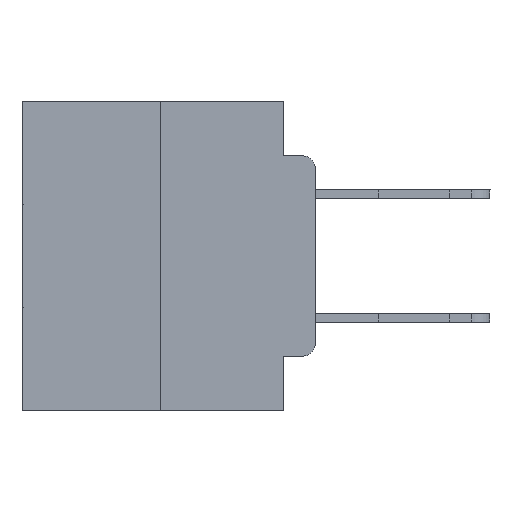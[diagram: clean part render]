
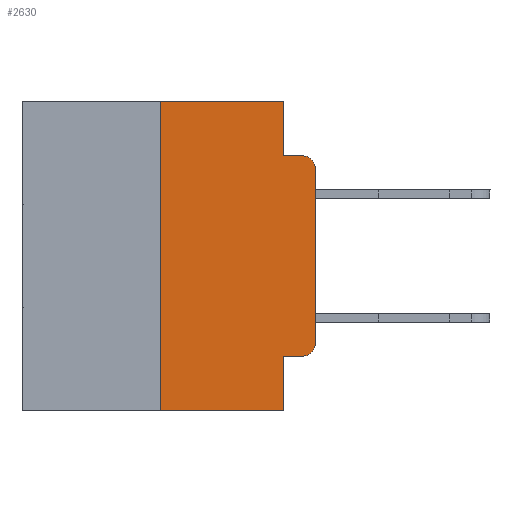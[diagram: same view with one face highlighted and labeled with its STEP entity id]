
A CAD part, left-side view. The second image highlights one B-rep face of the part: STEP entity #2630.
In plain terms, the highlighted planar face has unit normal (-1, 0, 0).
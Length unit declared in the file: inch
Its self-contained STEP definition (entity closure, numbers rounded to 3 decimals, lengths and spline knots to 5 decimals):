
#457 = ORIENTED_EDGE ( 'NONE', *, *, #23439, .T. ) ;
#731 = VERTEX_POINT ( 'NONE', #12477 ) ;
#1020 = CARTESIAN_POINT ( 'NONE',  ( 0., 0.02, -0.3915 ) ) ;
#1279 = EDGE_CURVE ( 'NONE', #29224, #14309, #18405, .T. ) ;
#1394 = VERTEX_POINT ( 'NONE', #22606 ) ;
#1662 = DIRECTION ( 'NONE',  ( 1., 0., 0. ) ) ;
#1730 = ORIENTED_EDGE ( 'NONE', *, *, #23288, .T. ) ;
#1739 = VECTOR ( 'NONE', #5891, 39.37008 ) ;
#2058 = FACE_OUTER_BOUND ( 'NONE', #27582, .T. ) ;
#2630 = ADVANCED_FACE ( 'NONE', ( #2058 ), #8108, .F. ) ;
#2900 = CARTESIAN_POINT ( 'NONE',  ( 0., 0.051, 0. ) ) ;
#3044 = LINE ( 'NONE', #14722, #4807 ) ;
#3130 = ORIENTED_EDGE ( 'NONE', *, *, #1279, .F. ) ;
#3200 = ORIENTED_EDGE ( 'NONE', *, *, #10787, .F. ) ;
#3272 = CARTESIAN_POINT ( 'NONE',  ( 0., 0., 0. ) ) ;
#3306 = DIRECTION ( 'NONE',  ( 0., 0., -1. ) ) ;
#3403 = DIRECTION ( 'NONE',  ( 0., -1., 0. ) ) ;
#3716 = VECTOR ( 'NONE', #18829, 39.37008 ) ;
#3768 = EDGE_CURVE ( 'NONE', #24552, #23078, #4485, .T. ) ;
#4485 = LINE ( 'NONE', #3272, #29301 ) ;
#4635 = VECTOR ( 'NONE', #11058, 39.37008 ) ;
#4807 = VECTOR ( 'NONE', #3403, 39.37008 ) ;
#4873 = LINE ( 'NONE', #20685, #14089 ) ;
#4961 = VERTEX_POINT ( 'NONE', #11347 ) ;
#5089 = CARTESIAN_POINT ( 'NONE',  ( 0., 0.25, 0. ) ) ;
#5126 = LINE ( 'NONE', #2900, #3716 ) ;
#5590 = CARTESIAN_POINT ( 'NONE',  ( 0., 0.051, 0. ) ) ;
#5891 = DIRECTION ( 'NONE',  ( 0., -1., 0. ) ) ;
#6029 = CARTESIAN_POINT ( 'NONE',  ( 0., 0.473, 0. ) ) ;
#6037 = VERTEX_POINT ( 'NONE', #10441 ) ;
#6317 = DIRECTION ( 'NONE',  ( 0., 0., -1. ) ) ;
#6622 = ORIENTED_EDGE ( 'NONE', *, *, #19904, .T. ) ;
#6926 = DIRECTION ( 'NONE',  ( 0., -1., 0. ) ) ;
#7267 = AXIS2_PLACEMENT_3D ( 'NONE', #1020, #19250, #3306 ) ;
#7724 = DIRECTION ( 'NONE',  ( 0., 0., -1. ) ) ;
#8108 = PLANE ( 'NONE',  #27756 ) ;
#9238 = LINE ( 'NONE', #22709, #4635 ) ;
#9262 = ORIENTED_EDGE ( 'NONE', *, *, #23024, .F. ) ;
#9304 = CARTESIAN_POINT ( 'NONE',  ( 0., 0., -0.3915 ) ) ;
#9660 = CARTESIAN_POINT ( 'NONE',  ( 0., 0.02, -0.1085 ) ) ;
#9723 = CARTESIAN_POINT ( 'NONE',  ( 0., 0.051, 0. ) ) ;
#9812 = VECTOR ( 'NONE', #17413, 39.37008 ) ;
#10441 = CARTESIAN_POINT ( 'NONE',  ( 0., 0.051, -0.5 ) ) ;
#10485 = CARTESIAN_POINT ( 'NONE',  ( 0., 0., -0.1085 ) ) ;
#10787 = EDGE_CURVE ( 'NONE', #14309, #4961, #5126, .T. ) ;
#11058 = DIRECTION ( 'NONE',  ( 0., -1., 0. ) ) ;
#11347 = CARTESIAN_POINT ( 'NONE',  ( 0., 0.051, -0.0885 ) ) ;
#11369 = EDGE_CURVE ( 'NONE', #4961, #1394, #4873, .T. ) ;
#11550 = CIRCLE ( 'NONE', #7267, 0.02 ) ;
#11762 = VERTEX_POINT ( 'NONE', #24329 ) ;
#12477 = CARTESIAN_POINT ( 'NONE',  ( 0., 0.02, -0.4115 ) ) ;
#12588 = ORIENTED_EDGE ( 'NONE', *, *, #23421, .T. ) ;
#14089 = VECTOR ( 'NONE', #6926, 39.37008 ) ;
#14309 = VERTEX_POINT ( 'NONE', #5590 ) ;
#14313 = AXIS2_PLACEMENT_3D ( 'NONE', #9660, #25477, #25290 ) ;
#14562 = CARTESIAN_POINT ( 'NONE',  ( 0., 0.051, -0.4115 ) ) ;
#14632 = CARTESIAN_POINT ( 'NONE',  ( 0., 0.473, 0. ) ) ;
#14722 = CARTESIAN_POINT ( 'NONE',  ( 0., 0.473, -0.5 ) ) ;
#15078 = ORIENTED_EDGE ( 'NONE', *, *, #11369, .F. ) ;
#15139 = CARTESIAN_POINT ( 'NONE',  ( 0., 0.25, 0. ) ) ;
#15762 = ORIENTED_EDGE ( 'NONE', *, *, #28300, .F. ) ;
#15861 = CIRCLE ( 'NONE', #14313, 0.02 ) ;
#17413 = DIRECTION ( 'NONE',  ( 0., 0., 1. ) ) ;
#17610 = VERTEX_POINT ( 'NONE', #14562 ) ;
#18405 = LINE ( 'NONE', #14632, #1739 ) ;
#18829 = DIRECTION ( 'NONE',  ( 0., 0., -1. ) ) ;
#19181 = VECTOR ( 'NONE', #7724, 39.37008 ) ;
#19250 = DIRECTION ( 'NONE',  ( -1., 0., 0. ) ) ;
#19904 = EDGE_CURVE ( 'NONE', #17610, #731, #9238, .T. ) ;
#20685 = CARTESIAN_POINT ( 'NONE',  ( 0., 0.051, -0.0885 ) ) ;
#22606 = CARTESIAN_POINT ( 'NONE',  ( 0., 0.02, -0.0885 ) ) ;
#22709 = CARTESIAN_POINT ( 'NONE',  ( 0., 0.051, -0.4115 ) ) ;
#22866 = ORIENTED_EDGE ( 'NONE', *, *, #3768, .T. ) ;
#23024 = EDGE_CURVE ( 'NONE', #11762, #29224, #25367, .T. ) ;
#23078 = VERTEX_POINT ( 'NONE', #10485 ) ;
#23288 = EDGE_CURVE ( 'NONE', #23078, #1394, #15861, .T. ) ;
#23421 = EDGE_CURVE ( 'NONE', #11762, #6037, #3044, .T. ) ;
#23439 = EDGE_CURVE ( 'NONE', #731, #24552, #11550, .T. ) ;
#23657 = DIRECTION ( 'NONE',  ( 0., 0., 1. ) ) ;
#24329 = CARTESIAN_POINT ( 'NONE',  ( 0., 0.25, -0.5 ) ) ;
#24552 = VERTEX_POINT ( 'NONE', #9304 ) ;
#24844 = LINE ( 'NONE', #9723, #19181 ) ;
#25290 = DIRECTION ( 'NONE',  ( 0., 0., -1. ) ) ;
#25367 = LINE ( 'NONE', #15139, #9812 ) ;
#25477 = DIRECTION ( 'NONE',  ( -1., 0., 0. ) ) ;
#27582 = EDGE_LOOP ( 'NONE', ( #22866, #1730, #15078, #3200, #3130, #9262, #12588, #15762, #6622, #457 ) ) ;
#27756 = AXIS2_PLACEMENT_3D ( 'NONE', #6029, #1662, #6317 ) ;
#28300 = EDGE_CURVE ( 'NONE', #17610, #6037, #24844, .T. ) ;
#29224 = VERTEX_POINT ( 'NONE', #5089 ) ;
#29301 = VECTOR ( 'NONE', #23657, 39.37008 ) ;
